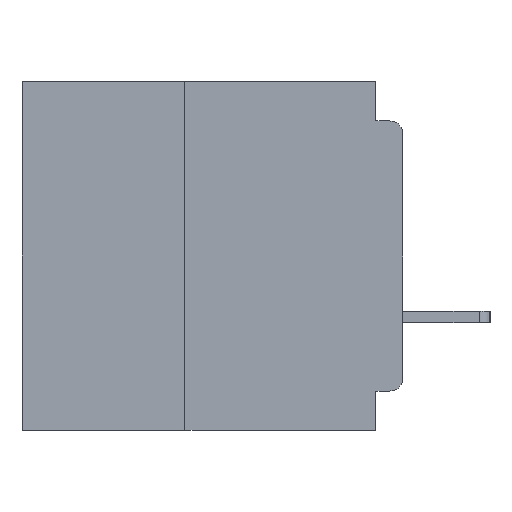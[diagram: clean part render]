
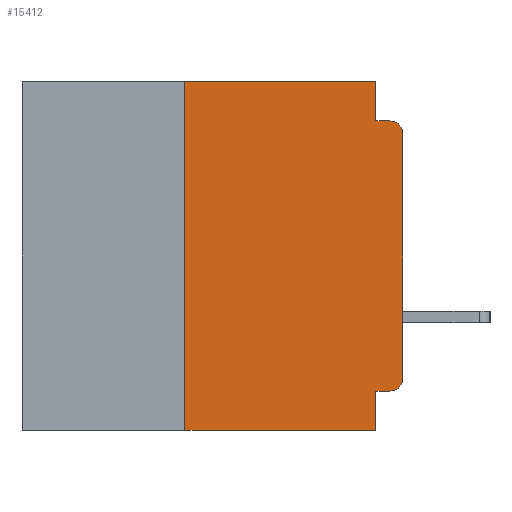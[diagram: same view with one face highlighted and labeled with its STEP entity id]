
A CAD part, left-side view. The second image highlights one B-rep face of the part: STEP entity #15412.
In plain terms, the highlighted planar face has unit normal (-1, 0, 0).
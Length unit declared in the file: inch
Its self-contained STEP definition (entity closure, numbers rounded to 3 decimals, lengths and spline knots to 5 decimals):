
#318 = VERTEX_POINT ( 'NONE', #38972 ) ;
#1073 = EDGE_CURVE ( 'NONE', #14389, #318, #33250, .T. ) ;
#1326 = VERTEX_POINT ( 'NONE', #24776 ) ;
#1523 = VECTOR ( 'NONE', #9181, 39.37008 ) ;
#1908 = VERTEX_POINT ( 'NONE', #13465 ) ;
#2095 = DIRECTION ( 'NONE',  ( 0., -1., 0. ) ) ;
#2132 = EDGE_CURVE ( 'NONE', #10922, #5012, #33654, .T. ) ;
#2143 = ORIENTED_EDGE ( 'NONE', *, *, #1073, .F. ) ;
#2242 = FACE_OUTER_BOUND ( 'NONE', #31913, .T. ) ;
#2457 = LINE ( 'NONE', #9620, #27804 ) ;
#2815 = DIRECTION ( 'NONE',  ( 0., 1., 0. ) ) ;
#3256 = CARTESIAN_POINT ( 'NONE',  ( 0., 0., -0.06 ) ) ;
#5012 = VERTEX_POINT ( 'NONE', #10684 ) ;
#5170 = ORIENTED_EDGE ( 'NONE', *, *, #37607, .F. ) ;
#6116 = AXIS2_PLACEMENT_3D ( 'NONE', #12518, #34629, #15744 ) ;
#6516 = EDGE_CURVE ( 'NONE', #1326, #8431, #10063, .T. ) ;
#7389 = CARTESIAN_POINT ( 'NONE',  ( 0., 0.25, -0.4 ) ) ;
#7725 = VECTOR ( 'NONE', #19989, 39.37008 ) ;
#8061 = DIRECTION ( 'NONE',  ( 0., 0., -1. ) ) ;
#8431 = VERTEX_POINT ( 'NONE', #3256 ) ;
#8650 = ORIENTED_EDGE ( 'NONE', *, *, #26547, .T. ) ;
#9181 = DIRECTION ( 'NONE',  ( 0., 0., 1. ) ) ;
#9620 = CARTESIAN_POINT ( 'NONE',  ( 0., 0., -0.045 ) ) ;
#10063 = LINE ( 'NONE', #15495, #1523 ) ;
#10300 = VERTEX_POINT ( 'NONE', #22749 ) ;
#10620 = EDGE_CURVE ( 'NONE', #20485, #10922, #27575, .T. ) ;
#10684 = CARTESIAN_POINT ( 'NONE',  ( 0., 0.031, -0.4 ) ) ;
#10922 = VERTEX_POINT ( 'NONE', #16903 ) ;
#11717 = CARTESIAN_POINT ( 'NONE',  ( 0., 0.015, -0.34 ) ) ;
#12518 = CARTESIAN_POINT ( 'NONE',  ( 0., 0.015, -0.06 ) ) ;
#13465 = CARTESIAN_POINT ( 'NONE',  ( 0., 0.25, 0. ) ) ;
#14368 = CARTESIAN_POINT ( 'NONE',  ( 0., 0.437, 0. ) ) ;
#14389 = VERTEX_POINT ( 'NONE', #21885 ) ;
#14953 = DIRECTION ( 'NONE',  ( 0., 0., -1. ) ) ;
#15412 = ADVANCED_FACE ( 'NONE', ( #2242 ), #36442, .F. ) ;
#15495 = CARTESIAN_POINT ( 'NONE',  ( 0., 0., 0. ) ) ;
#15744 = DIRECTION ( 'NONE',  ( 0., 0., -1. ) ) ;
#15745 = AXIS2_PLACEMENT_3D ( 'NONE', #14368, #27048, #8061 ) ;
#16137 = ORIENTED_EDGE ( 'NONE', *, *, #21700, .F. ) ;
#16150 = ORIENTED_EDGE ( 'NONE', *, *, #30389, .T. ) ;
#16751 = CIRCLE ( 'NONE', #6116, 0.015 ) ;
#16821 = CARTESIAN_POINT ( 'NONE',  ( 0., 0.437, -0.4 ) ) ;
#16882 = VECTOR ( 'NONE', #18817, 39.37008 ) ;
#16903 = CARTESIAN_POINT ( 'NONE',  ( 0., 0.031, -0.355 ) ) ;
#16961 = VECTOR ( 'NONE', #2095, 39.37008 ) ;
#17983 = CARTESIAN_POINT ( 'NONE',  ( 0., 0.437, 0. ) ) ;
#18817 = DIRECTION ( 'NONE',  ( 0., 0., -1. ) ) ;
#19662 = CIRCLE ( 'NONE', #36036, 0.015 ) ;
#19989 = DIRECTION ( 'NONE',  ( 0., -1., 0. ) ) ;
#20485 = VERTEX_POINT ( 'NONE', #33396 ) ;
#20691 = CARTESIAN_POINT ( 'NONE',  ( 0., 0.031, 0. ) ) ;
#21700 = EDGE_CURVE ( 'NONE', #1908, #14389, #26351, .T. ) ;
#21885 = CARTESIAN_POINT ( 'NONE',  ( 0., 0.031, 0. ) ) ;
#22749 = CARTESIAN_POINT ( 'NONE',  ( 0., 0.25, -0.4 ) ) ;
#23203 = LINE ( 'NONE', #7389, #39973 ) ;
#23222 = DIRECTION ( 'NONE',  ( 0., 0., 1. ) ) ;
#23609 = ORIENTED_EDGE ( 'NONE', *, *, #6516, .T. ) ;
#24674 = DIRECTION ( 'NONE',  ( 0., 0., -1. ) ) ;
#24776 = CARTESIAN_POINT ( 'NONE',  ( 0., 0., -0.34 ) ) ;
#24876 = VECTOR ( 'NONE', #24674, 39.37008 ) ;
#25071 = CARTESIAN_POINT ( 'NONE',  ( 0., 0., -0.355 ) ) ;
#25948 = EDGE_CURVE ( 'NONE', #10300, #1908, #23203, .T. ) ;
#26315 = EDGE_CURVE ( 'NONE', #8431, #39498, #16751, .T. ) ;
#26351 = LINE ( 'NONE', #17983, #16961 ) ;
#26524 = ORIENTED_EDGE ( 'NONE', *, *, #25948, .F. ) ;
#26547 = EDGE_CURVE ( 'NONE', #10300, #5012, #32988, .T. ) ;
#26607 = VECTOR ( 'NONE', #2815, 39.37008 ) ;
#27048 = DIRECTION ( 'NONE',  ( 1., 0., 0. ) ) ;
#27575 = LINE ( 'NONE', #25071, #26607 ) ;
#27804 = VECTOR ( 'NONE', #31749, 39.37008 ) ;
#28192 = CARTESIAN_POINT ( 'NONE',  ( 0., 0.031, -0.4 ) ) ;
#30389 = EDGE_CURVE ( 'NONE', #20485, #1326, #19662, .T. ) ;
#31749 = DIRECTION ( 'NONE',  ( 0., -1., 0. ) ) ;
#31913 = EDGE_LOOP ( 'NONE', ( #23609, #39335, #5170, #2143, #16137, #26524, #8650, #33898, #32922, #16150 ) ) ;
#32922 = ORIENTED_EDGE ( 'NONE', *, *, #10620, .F. ) ;
#32988 = LINE ( 'NONE', #16821, #7725 ) ;
#33250 = LINE ( 'NONE', #20691, #24876 ) ;
#33396 = CARTESIAN_POINT ( 'NONE',  ( 0., 0.015, -0.355 ) ) ;
#33654 = LINE ( 'NONE', #28192, #16882 ) ;
#33844 = DIRECTION ( 'NONE',  ( -1., 0., 0. ) ) ;
#33898 = ORIENTED_EDGE ( 'NONE', *, *, #2132, .F. ) ;
#34629 = DIRECTION ( 'NONE',  ( -1., 0., 0. ) ) ;
#36036 = AXIS2_PLACEMENT_3D ( 'NONE', #11717, #33844, #14953 ) ;
#36442 = PLANE ( 'NONE',  #15745 ) ;
#37607 = EDGE_CURVE ( 'NONE', #318, #39498, #2457, .T. ) ;
#38972 = CARTESIAN_POINT ( 'NONE',  ( 0., 0.031, -0.045 ) ) ;
#39335 = ORIENTED_EDGE ( 'NONE', *, *, #26315, .T. ) ;
#39498 = VERTEX_POINT ( 'NONE', #40293 ) ;
#39973 = VECTOR ( 'NONE', #23222, 39.37008 ) ;
#40293 = CARTESIAN_POINT ( 'NONE',  ( 0., 0.015, -0.045 ) ) ;
